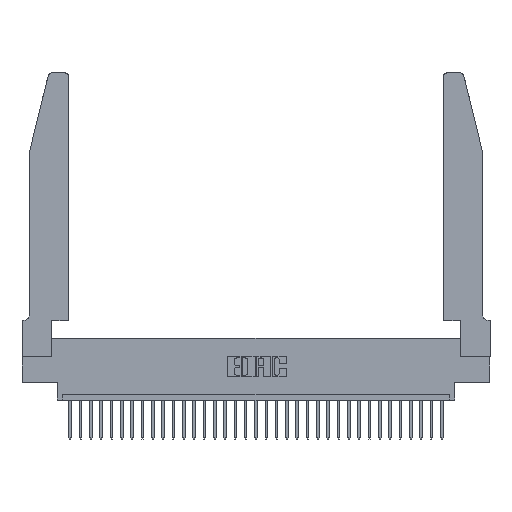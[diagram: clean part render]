
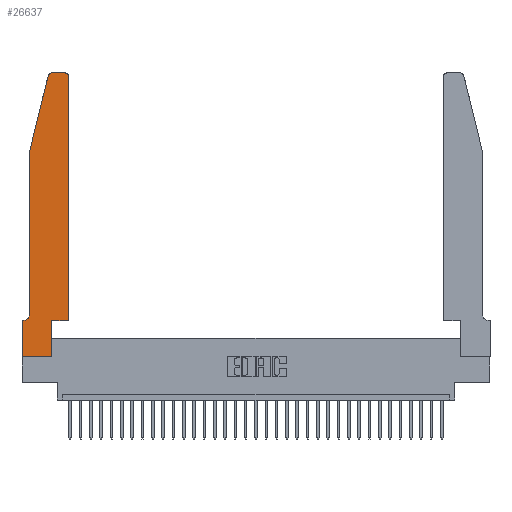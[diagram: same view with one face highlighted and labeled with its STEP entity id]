
A CAD part, top view. The second image highlights one B-rep face of the part: STEP entity #26637.
In plain terms, the highlighted planar face has unit normal (0, 0, 1).
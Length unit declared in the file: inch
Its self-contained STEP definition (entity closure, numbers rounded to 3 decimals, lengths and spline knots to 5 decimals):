
#256 = LINE ( 'NONE', #8801, #21278 ) ;
#479 = VERTEX_POINT ( 'NONE', #17054 ) ;
#736 = DIRECTION ( 'NONE',  ( 1., 0., 0. ) ) ;
#740 = VERTEX_POINT ( 'NONE', #4885 ) ;
#992 = FACE_OUTER_BOUND ( 'NONE', #14964, .T. ) ;
#1143 = CIRCLE ( 'NONE', #3930, 0.07 ) ;
#1280 = EDGE_CURVE ( 'NONE', #479, #21091, #29852, .T. ) ;
#1733 = DIRECTION ( 'NONE',  ( -1., 0., 0. ) ) ;
#2255 = DIRECTION ( 'NONE',  ( 0., -1., 0. ) ) ;
#3447 = EDGE_CURVE ( 'NONE', #740, #21528, #12833, .T. ) ;
#3702 = VERTEX_POINT ( 'NONE', #7249 ) ;
#3791 = ORIENTED_EDGE ( 'NONE', *, *, #24018, .T. ) ;
#3930 = AXIS2_PLACEMENT_3D ( 'NONE', #13966, #8993, #16738 ) ;
#3984 = VECTOR ( 'NONE', #5718, 39.37008 ) ;
#4573 = VERTEX_POINT ( 'NONE', #10682 ) ;
#4656 = ORIENTED_EDGE ( 'NONE', *, *, #18379, .T. ) ;
#4801 = EDGE_CURVE ( 'NONE', #3702, #4573, #1143, .T. ) ;
#4885 = CARTESIAN_POINT ( 'NONE',  ( 0.284, 2.75, 0.37 ) ) ;
#5211 = ORIENTED_EDGE ( 'NONE', *, *, #1280, .T. ) ;
#5718 = DIRECTION ( 'NONE',  ( -0.239, -0.971, 0. ) ) ;
#5850 = VECTOR ( 'NONE', #1733, 39.37008 ) ;
#5958 = CARTESIAN_POINT ( 'NONE',  ( 0.0755, 2., 0.37 ) ) ;
#6059 = CARTESIAN_POINT ( 'NONE',  ( 0.4205, 2.72, 0.37 ) ) ;
#6551 = VECTOR ( 'NONE', #18476, 39.37008 ) ;
#6686 = CARTESIAN_POINT ( 'NONE',  ( 0., 0.35, 0.37 ) ) ;
#6961 = VECTOR ( 'NONE', #7279, 39.37008 ) ;
#7249 = CARTESIAN_POINT ( 'NONE',  ( 0.0755, 0.42, 0.37 ) ) ;
#7279 = DIRECTION ( 'NONE',  ( 0., 1., 0. ) ) ;
#7483 = AXIS2_PLACEMENT_3D ( 'NONE', #6059, #26419, #736 ) ;
#7596 = LINE ( 'NONE', #5958, #3984 ) ;
#7828 = CARTESIAN_POINT ( 'NONE',  ( 0.0755, 2., 0.37 ) ) ;
#8801 = CARTESIAN_POINT ( 'NONE',  ( 0., 0., 0.37 ) ) ;
#8912 = DIRECTION ( 'NONE',  ( 1., 0., 0. ) ) ;
#8993 = DIRECTION ( 'NONE',  ( 0., 0., -1. ) ) ;
#9535 = CARTESIAN_POINT ( 'NONE',  ( 0.2865, 0., 0.37 ) ) ;
#10682 = CARTESIAN_POINT ( 'NONE',  ( 0.0055, 0.35, 0.37 ) ) ;
#11156 = EDGE_CURVE ( 'NONE', #19598, #479, #23060, .T. ) ;
#11385 = VERTEX_POINT ( 'NONE', #15575 ) ;
#12189 = CARTESIAN_POINT ( 'NONE',  ( 0.4505, 0.35, 0.37 ) ) ;
#12260 = LINE ( 'NONE', #17450, #18732 ) ;
#12486 = AXIS2_PLACEMENT_3D ( 'NONE', #28649, #23433, #18270 ) ;
#12833 = CIRCLE ( 'NONE', #12486, 0.03 ) ;
#12903 = EDGE_CURVE ( 'NONE', #19117, #3702, #27014, .T. ) ;
#13081 = CARTESIAN_POINT ( 'NONE',  ( 0., 0., 0.37 ) ) ;
#13545 = VERTEX_POINT ( 'NONE', #31586 ) ;
#13896 = VERTEX_POINT ( 'NONE', #14188 ) ;
#13966 = CARTESIAN_POINT ( 'NONE',  ( 0.0055, 0.42, 0.37 ) ) ;
#14188 = CARTESIAN_POINT ( 'NONE',  ( 0.4205, 2.75, 0.37 ) ) ;
#14292 = ORIENTED_EDGE ( 'NONE', *, *, #16938, .T. ) ;
#14537 = DIRECTION ( 'NONE',  ( 0., 0., 1. ) ) ;
#14964 = EDGE_LOOP ( 'NONE', ( #4656, #27218, #14292, #20001, #29863, #17453, #19627, #17716, #16284, #5211, #3791, #23764 ) ) ;
#15575 = CARTESIAN_POINT ( 'NONE',  ( 0.4505, 2.72, 0.37 ) ) ;
#16275 = CARTESIAN_POINT ( 'NONE',  ( 0.2605, 2.75, 0.37 ) ) ;
#16284 = ORIENTED_EDGE ( 'NONE', *, *, #11156, .T. ) ;
#16738 = DIRECTION ( 'NONE',  ( -1., 0., 0. ) ) ;
#16938 = EDGE_CURVE ( 'NONE', #21528, #19117, #7596, .T. ) ;
#17054 = CARTESIAN_POINT ( 'NONE',  ( 0.2865, 0.35, 0.37 ) ) ;
#17450 = CARTESIAN_POINT ( 'NONE',  ( 0.4505, 0.35, 0.37 ) ) ;
#17453 = ORIENTED_EDGE ( 'NONE', *, *, #28231, .T. ) ;
#17545 = EDGE_CURVE ( 'NONE', #22534, #19598, #256, .T. ) ;
#17716 = ORIENTED_EDGE ( 'NONE', *, *, #17545, .T. ) ;
#17830 = CARTESIAN_POINT ( 'NONE',  ( 0., 0., 0.37 ) ) ;
#17975 = CARTESIAN_POINT ( 'NONE',  ( 0.2865, 0.35, 0.37 ) ) ;
#18270 = DIRECTION ( 'NONE',  ( 1., 0., 0. ) ) ;
#18379 = EDGE_CURVE ( 'NONE', #13896, #740, #27350, .T. ) ;
#18476 = DIRECTION ( 'NONE',  ( 0., -1., 0. ) ) ;
#18732 = VECTOR ( 'NONE', #20276, 39.37008 ) ;
#19117 = VERTEX_POINT ( 'NONE', #7828 ) ;
#19484 = PLANE ( 'NONE',  #24646 ) ;
#19598 = VERTEX_POINT ( 'NONE', #9535 ) ;
#19627 = ORIENTED_EDGE ( 'NONE', *, *, #26283, .T. ) ;
#20001 = ORIENTED_EDGE ( 'NONE', *, *, #12903, .T. ) ;
#20139 = VECTOR ( 'NONE', #2255, 39.37008 ) ;
#20276 = DIRECTION ( 'NONE',  ( 0., 1., 0. ) ) ;
#20475 = VECTOR ( 'NONE', #24930, 39.37008 ) ;
#21091 = VERTEX_POINT ( 'NONE', #12189 ) ;
#21278 = VECTOR ( 'NONE', #8912, 39.37008 ) ;
#21528 = VERTEX_POINT ( 'NONE', #26162 ) ;
#22534 = VERTEX_POINT ( 'NONE', #17830 ) ;
#22938 = CIRCLE ( 'NONE', #7483, 0.03 ) ;
#23060 = LINE ( 'NONE', #17975, #6961 ) ;
#23125 = DIRECTION ( 'NONE',  ( 1., 0., 0. ) ) ;
#23433 = DIRECTION ( 'NONE',  ( 0., 0., 1. ) ) ;
#23764 = ORIENTED_EDGE ( 'NONE', *, *, #32234, .T. ) ;
#24018 = EDGE_CURVE ( 'NONE', #21091, #11385, #12260, .T. ) ;
#24646 = AXIS2_PLACEMENT_3D ( 'NONE', #6686, #14537, #32621 ) ;
#24648 = LINE ( 'NONE', #13081, #6551 ) ;
#24930 = DIRECTION ( 'NONE',  ( -1., 0., 0. ) ) ;
#26000 = LINE ( 'NONE', #32646, #5850 ) ;
#26162 = CARTESIAN_POINT ( 'NONE',  ( 0.25487, 2.72718, 0.37 ) ) ;
#26283 = EDGE_CURVE ( 'NONE', #13545, #22534, #24648, .T. ) ;
#26419 = DIRECTION ( 'NONE',  ( 0., 0., 1. ) ) ;
#26637 = ADVANCED_FACE ( 'NONE', ( #992 ), #19484, .T. ) ;
#27014 = LINE ( 'NONE', #30453, #20139 ) ;
#27218 = ORIENTED_EDGE ( 'NONE', *, *, #3447, .T. ) ;
#27350 = LINE ( 'NONE', #16275, #20475 ) ;
#28138 = CARTESIAN_POINT ( 'NONE',  ( 0.4505, 0.35, 0.37 ) ) ;
#28231 = EDGE_CURVE ( 'NONE', #4573, #13545, #26000, .T. ) ;
#28649 = CARTESIAN_POINT ( 'NONE',  ( 0.284, 2.72, 0.37 ) ) ;
#29002 = VECTOR ( 'NONE', #23125, 39.37008 ) ;
#29852 = LINE ( 'NONE', #28138, #29002 ) ;
#29863 = ORIENTED_EDGE ( 'NONE', *, *, #4801, .T. ) ;
#30453 = CARTESIAN_POINT ( 'NONE',  ( 0.0755, 2., 0.37 ) ) ;
#31586 = CARTESIAN_POINT ( 'NONE',  ( 0., 0.35, 0.37 ) ) ;
#32234 = EDGE_CURVE ( 'NONE', #11385, #13896, #22938, .T. ) ;
#32621 = DIRECTION ( 'NONE',  ( 1., 0., 0. ) ) ;
#32646 = CARTESIAN_POINT ( 'NONE',  ( 0.0755, 0.35, 0.37 ) ) ;
